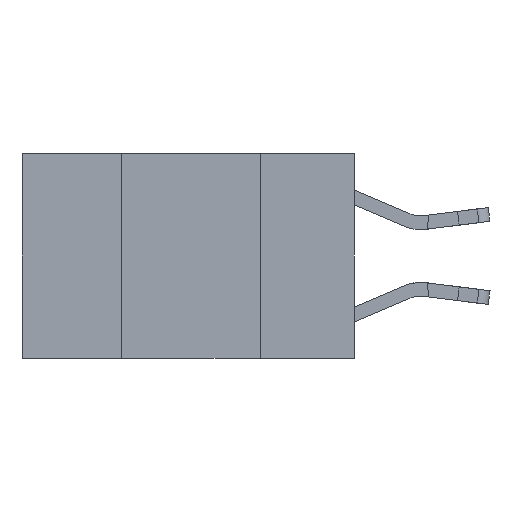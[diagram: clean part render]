
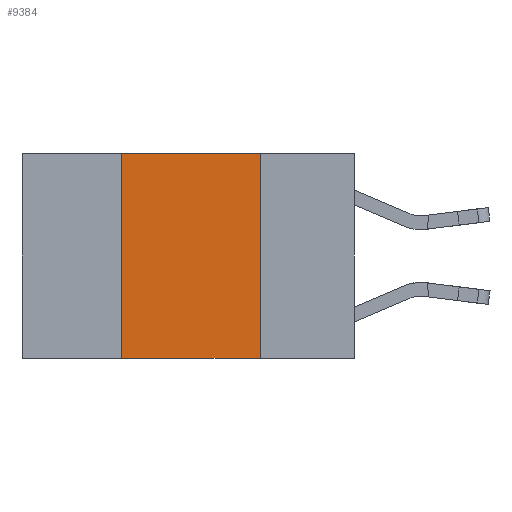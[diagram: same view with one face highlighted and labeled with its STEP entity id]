
A CAD part, left-side view. The second image highlights one B-rep face of the part: STEP entity #9384.
In plain terms, the highlighted planar face has unit normal (-1, 0, 0).
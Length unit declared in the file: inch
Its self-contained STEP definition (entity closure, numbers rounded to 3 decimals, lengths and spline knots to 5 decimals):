
#654 = ORIENTED_EDGE ( 'NONE', *, *, #21809, .F. ) ;
#1949 = VERTEX_POINT ( 'NONE', #2926 ) ;
#2242 = ORIENTED_EDGE ( 'NONE', *, *, #16546, .T. ) ;
#2926 = CARTESIAN_POINT ( 'NONE',  ( 0., 0.42, 0. ) ) ;
#3469 = FACE_OUTER_BOUND ( 'NONE', #25156, .T. ) ;
#3668 = DIRECTION ( 'NONE',  ( 0., 0., -1. ) ) ;
#4036 = VECTOR ( 'NONE', #25632, 39.37008 ) ;
#4162 = ORIENTED_EDGE ( 'NONE', *, *, #19528, .F. ) ;
#5774 = DIRECTION ( 'NONE',  ( 0., 0., -1. ) ) ;
#9076 = LINE ( 'NONE', #17018, #21662 ) ;
#9384 = ADVANCED_FACE ( 'NONE', ( #3469 ), #16963, .F. ) ;
#10527 = VERTEX_POINT ( 'NONE', #15245 ) ;
#12567 = CARTESIAN_POINT ( 'NONE',  ( 0., 0.6, -0.37 ) ) ;
#15227 = LINE ( 'NONE', #23527, #4036 ) ;
#15245 = CARTESIAN_POINT ( 'NONE',  ( 0., 0.42, -0.37 ) ) ;
#16546 = EDGE_CURVE ( 'NONE', #10527, #17363, #27723, .T. ) ;
#16909 = VECTOR ( 'NONE', #27778, 39.37008 ) ;
#16963 = PLANE ( 'NONE',  #23592 ) ;
#17018 = CARTESIAN_POINT ( 'NONE',  ( 0., 0.17, 0. ) ) ;
#17363 = VERTEX_POINT ( 'NONE', #24064 ) ;
#17684 = DIRECTION ( 'NONE',  ( 0., 0., 1. ) ) ;
#18040 = EDGE_CURVE ( 'NONE', #10527, #1949, #22365, .T. ) ;
#19195 = DIRECTION ( 'NONE',  ( 1., 0., 0. ) ) ;
#19528 = EDGE_CURVE ( 'NONE', #21239, #17363, #9076, .T. ) ;
#21239 = VERTEX_POINT ( 'NONE', #21307 ) ;
#21307 = CARTESIAN_POINT ( 'NONE',  ( 0., 0.17, 0. ) ) ;
#21662 = VECTOR ( 'NONE', #3668, 39.37008 ) ;
#21809 = EDGE_CURVE ( 'NONE', #1949, #21239, #15227, .T. ) ;
#22365 = LINE ( 'NONE', #24288, #27301 ) ;
#23505 = CARTESIAN_POINT ( 'NONE',  ( 0., 0.6, 0. ) ) ;
#23527 = CARTESIAN_POINT ( 'NONE',  ( 0., 0.6, 0. ) ) ;
#23592 = AXIS2_PLACEMENT_3D ( 'NONE', #23505, #19195, #5774 ) ;
#24064 = CARTESIAN_POINT ( 'NONE',  ( 0., 0.17, -0.37 ) ) ;
#24288 = CARTESIAN_POINT ( 'NONE',  ( 0., 0.42, 0. ) ) ;
#25156 = EDGE_LOOP ( 'NONE', ( #4162, #654, #27943, #2242 ) ) ;
#25632 = DIRECTION ( 'NONE',  ( 0., -1., 0. ) ) ;
#27301 = VECTOR ( 'NONE', #17684, 39.37008 ) ;
#27723 = LINE ( 'NONE', #12567, #16909 ) ;
#27778 = DIRECTION ( 'NONE',  ( 0., -1., 0. ) ) ;
#27943 = ORIENTED_EDGE ( 'NONE', *, *, #18040, .F. ) ;
